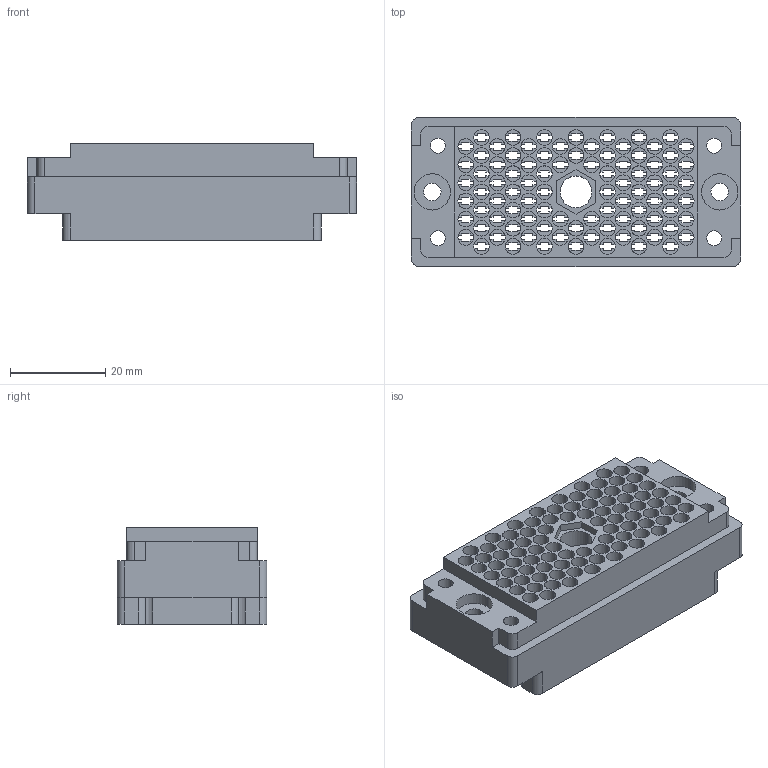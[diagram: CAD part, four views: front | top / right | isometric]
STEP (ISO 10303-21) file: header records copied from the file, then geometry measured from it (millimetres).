
FILE_DESCRIPTION (( 'STEP AP203' ), '1' );
FILE_NAME ('516-090-000-300.STEP', '2020-03-10T15:52:55', ( '' ), ( '' ), 'SwSTEP 2.0', 'SolidWorks 2016', '' );
FILE_SCHEMA (( 'CONFIG_CONTROL_DESIGN' ));
Length unit declared in the file: inch
Products named in the file (2): 516-090-000-300; 516 Plug Insulator_090
Assembly tree (1 placements, depth 2):
  516-090-000-300
    516 Plug Insulator_090
Bounding box: 69.04 x 31.34 x 20.27 mm (x, y, z)
Volume: 16708.2 mm3; surface area: 22126.1 mm2
Topology: 1 solids, 1 shells, 1846 faces, 5492 edges, 3660 vertices
Faces by surface type: plane 1383, cylinder 461, cone 2
Entity records: 62442 total; most frequent: CARTESIAN_POINT 11002, ORIENTED_EDGE 10984, DIRECTION 10482, EDGE_CURVE 5492, LINE 4202, VECTOR 4202, VERTEX_POINT 3660, AXIS2_PLACEMENT_3D 3140
